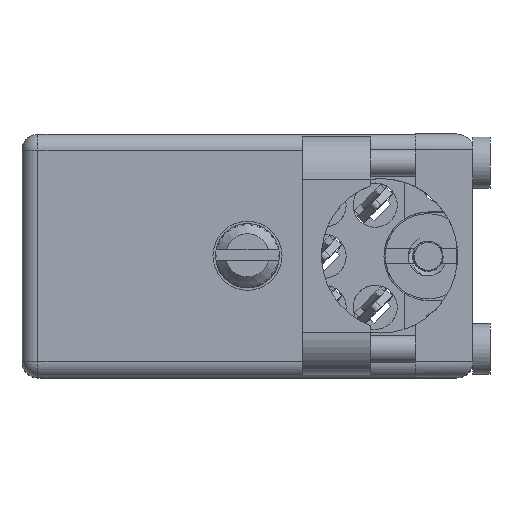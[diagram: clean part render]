
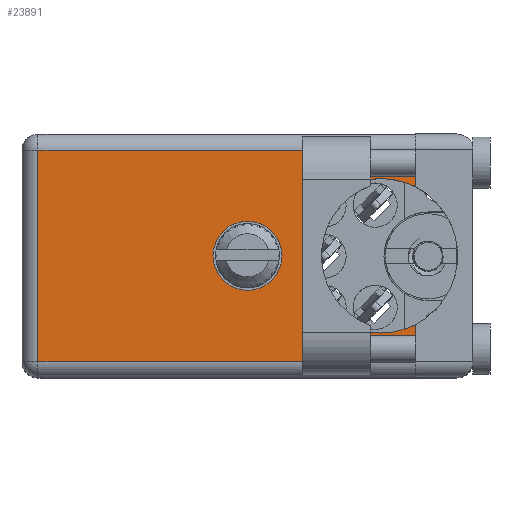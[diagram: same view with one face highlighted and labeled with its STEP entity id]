
A CAD part, top view. The second image highlights one B-rep face of the part: STEP entity #23891.
In plain terms, the highlighted face is planar.
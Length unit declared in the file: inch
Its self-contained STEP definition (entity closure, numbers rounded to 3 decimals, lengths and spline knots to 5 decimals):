
#274 = FACE_BOUND ( 'NONE', #188895, .T. ) ;
#8035 = CIRCLE ( 'NONE', #20502, 0.227 ) ;
#8631 = EDGE_CURVE ( 'NONE', #19854, #137624, #150939, .T. ) ;
#9552 = AXIS2_PLACEMENT_3D ( 'NONE', #80948, #142836, #124238 ) ;
#12812 = VECTOR ( 'NONE', #153067, 39.37008 ) ;
#13189 = VECTOR ( 'NONE', #136208, 39.37008 ) ;
#18637 = EDGE_CURVE ( 'NONE', #156800, #189742, #106875, .T. ) ;
#19854 = VERTEX_POINT ( 'NONE', #174503 ) ;
#20502 = AXIS2_PLACEMENT_3D ( 'NONE', #179450, #139157, #91020 ) ;
#21814 = CARTESIAN_POINT ( 'NONE',  ( 0.6625, 0.906, -0.3575 ) ) ;
#23375 = VERTEX_POINT ( 'NONE', #75332 ) ;
#23689 = DIRECTION ( 'NONE',  ( 0., 1., 0. ) ) ;
#23891 = ADVANCED_FACE ( 'NONE', ( #74872, #274 ), #60190, .T. ) ;
#26484 = EDGE_CURVE ( 'NONE', #189742, #137624, #115553, .T. ) ;
#30390 = CARTESIAN_POINT ( 'NONE',  ( 1.053, 0.906, -0.3575 ) ) ;
#31936 = CARTESIAN_POINT ( 'NONE',  ( 1.053, 0.906, -0.3575 ) ) ;
#37177 = AXIS2_PLACEMENT_3D ( 'NONE', #143527, #23689, #51263 ) ;
#41383 = EDGE_CURVE ( 'NONE', #23375, #19854, #187594, .T. ) ;
#41730 = CARTESIAN_POINT ( 'NONE',  ( 1.155, 0.906, -0.668 ) ) ;
#44999 = LINE ( 'NONE', #46930, #59353 ) ;
#46715 = DIRECTION ( 'NONE',  ( 0., 0., 1. ) ) ;
#46930 = CARTESIAN_POINT ( 'NONE',  ( 1.155, 0.906, 0. ) ) ;
#47503 = VERTEX_POINT ( 'NONE', #52339 ) ;
#49609 = CARTESIAN_POINT ( 'NONE',  ( 1.155, 0.906, -0.047 ) ) ;
#51263 = DIRECTION ( 'NONE',  ( 0., 0., 1. ) ) ;
#52339 = CARTESIAN_POINT ( 'NONE',  ( 0.6625, 0.906, -0.459 ) ) ;
#55173 = ORIENTED_EDGE ( 'NONE', *, *, #150384, .T. ) ;
#56671 = CARTESIAN_POINT ( 'NONE',  ( 1.155, 0.906, -0.047 ) ) ;
#59353 = VECTOR ( 'NONE', #167678, 39.37008 ) ;
#60190 = PLANE ( 'NONE',  #37177 ) ;
#66402 = ORIENTED_EDGE ( 'NONE', *, *, #26484, .T. ) ;
#67319 = VERTEX_POINT ( 'NONE', #41730 ) ;
#74502 = EDGE_LOOP ( 'NONE', ( #154792, #55173, #103285, #66402, #132892, #193049, #190986, #173924 ) ) ;
#74872 = FACE_OUTER_BOUND ( 'NONE', #74502, .T. ) ;
#75332 = CARTESIAN_POINT ( 'NONE',  ( 1.053, 0.906, -0.1305 ) ) ;
#78552 = VERTEX_POINT ( 'NONE', #189242 ) ;
#79292 = CARTESIAN_POINT ( 'NONE',  ( 1.155, 0.906, -0.56029 ) ) ;
#80023 = ORIENTED_EDGE ( 'NONE', *, *, #182413, .F. ) ;
#80948 = CARTESIAN_POINT ( 'NONE',  ( 0.6625, 0.906, -0.3575 ) ) ;
#82261 = VERTEX_POINT ( 'NONE', #79292 ) ;
#88751 = CARTESIAN_POINT ( 'NONE',  ( 0.047, 0.906, -0.668 ) ) ;
#90845 = DIRECTION ( 'NONE',  ( 0., 1., 0. ) ) ;
#91020 = DIRECTION ( 'NONE',  ( 0., 0., 1. ) ) ;
#93103 = CARTESIAN_POINT ( 'NONE',  ( 0.047, 0.906, -0.715 ) ) ;
#93938 = CARTESIAN_POINT ( 'NONE',  ( 0.047, 0.906, -0.047 ) ) ;
#100364 = CIRCLE ( 'NONE', #144308, 0.1015 ) ;
#102908 = AXIS2_PLACEMENT_3D ( 'NONE', #31936, #90845, #46715 ) ;
#103285 = ORIENTED_EDGE ( 'NONE', *, *, #18637, .T. ) ;
#106875 = LINE ( 'NONE', #93103, #12812 ) ;
#107640 = CARTESIAN_POINT ( 'NONE',  ( 1.155, 0.906, 0. ) ) ;
#107799 = DIRECTION ( 'NONE',  ( -1., 0., 0. ) ) ;
#110216 = DIRECTION ( 'NONE',  ( 0., 1., 0. ) ) ;
#114579 = DIRECTION ( 'NONE',  ( 1., 0., 0. ) ) ;
#115553 = LINE ( 'NONE', #56671, #159863 ) ;
#116100 = CIRCLE ( 'NONE', #9552, 0.1015 ) ;
#124238 = DIRECTION ( 'NONE',  ( 0., 0., 1. ) ) ;
#130422 = AXIS2_PLACEMENT_3D ( 'NONE', #30390, #167843, #134536 ) ;
#132892 = ORIENTED_EDGE ( 'NONE', *, *, #8631, .F. ) ;
#134536 = DIRECTION ( 'NONE',  ( 0., 0., 1. ) ) ;
#136208 = DIRECTION ( 'NONE',  ( 0., 0., 1. ) ) ;
#137624 = VERTEX_POINT ( 'NONE', #49609 ) ;
#138683 = VECTOR ( 'NONE', #107799, 39.37008 ) ;
#139157 = DIRECTION ( 'NONE',  ( 0., 1., 0. ) ) ;
#142268 = CARTESIAN_POINT ( 'NONE',  ( 1.053, 0.906, -0.5845 ) ) ;
#142836 = DIRECTION ( 'NONE',  ( 0., 1., 0. ) ) ;
#143527 = CARTESIAN_POINT ( 'NONE',  ( 0., 0.906, -0.715 ) ) ;
#144308 = AXIS2_PLACEMENT_3D ( 'NONE', #21814, #110216, #170145 ) ;
#150384 = EDGE_CURVE ( 'NONE', #67319, #156800, #152061, .T. ) ;
#150939 = LINE ( 'NONE', #107640, #13189 ) ;
#152061 = LINE ( 'NONE', #165835, #138683 ) ;
#153067 = DIRECTION ( 'NONE',  ( 0., 0., 1. ) ) ;
#154792 = ORIENTED_EDGE ( 'NONE', *, *, #173817, .F. ) ;
#154990 = EDGE_CURVE ( 'NONE', #172813, #23375, #8035, .T. ) ;
#156800 = VERTEX_POINT ( 'NONE', #88751 ) ;
#158700 = EDGE_CURVE ( 'NONE', #82261, #172813, #189992, .T. ) ;
#159863 = VECTOR ( 'NONE', #114579, 39.37008 ) ;
#165835 = CARTESIAN_POINT ( 'NONE',  ( 0., 0.906, -0.668 ) ) ;
#167678 = DIRECTION ( 'NONE',  ( 0., 0., 1. ) ) ;
#167843 = DIRECTION ( 'NONE',  ( 0., 1., 0. ) ) ;
#170145 = DIRECTION ( 'NONE',  ( 0., 0., 1. ) ) ;
#172813 = VERTEX_POINT ( 'NONE', #142268 ) ;
#173817 = EDGE_CURVE ( 'NONE', #67319, #82261, #44999, .T. ) ;
#173924 = ORIENTED_EDGE ( 'NONE', *, *, #158700, .F. ) ;
#174503 = CARTESIAN_POINT ( 'NONE',  ( 1.155, 0.906, -0.15471 ) ) ;
#179222 = EDGE_CURVE ( 'NONE', #78552, #47503, #100364, .T. ) ;
#179450 = CARTESIAN_POINT ( 'NONE',  ( 1.053, 0.906, -0.3575 ) ) ;
#179869 = ORIENTED_EDGE ( 'NONE', *, *, #179222, .F. ) ;
#182413 = EDGE_CURVE ( 'NONE', #47503, #78552, #116100, .T. ) ;
#187594 = CIRCLE ( 'NONE', #102908, 0.227 ) ;
#188895 = EDGE_LOOP ( 'NONE', ( #179869, #80023 ) ) ;
#189242 = CARTESIAN_POINT ( 'NONE',  ( 0.6625, 0.906, -0.256 ) ) ;
#189742 = VERTEX_POINT ( 'NONE', #93938 ) ;
#189992 = CIRCLE ( 'NONE', #130422, 0.227 ) ;
#190986 = ORIENTED_EDGE ( 'NONE', *, *, #154990, .F. ) ;
#193049 = ORIENTED_EDGE ( 'NONE', *, *, #41383, .F. ) ;
